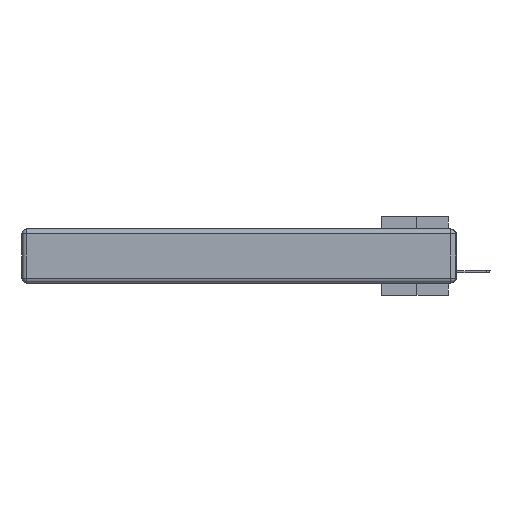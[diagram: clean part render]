
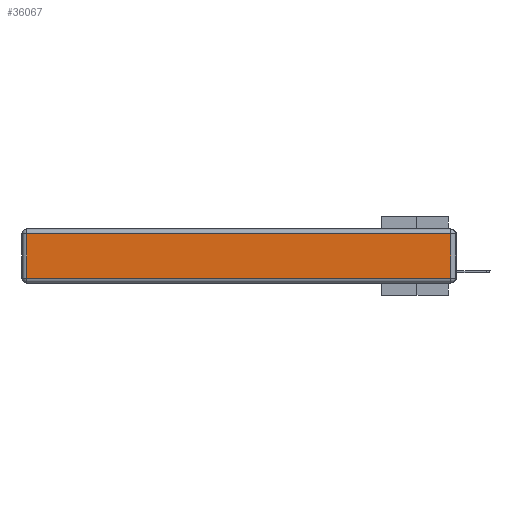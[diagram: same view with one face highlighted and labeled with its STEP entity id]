
A CAD part, left-side view. The second image highlights one B-rep face of the part: STEP entity #36067.
In plain terms, the highlighted planar face has unit normal (-1, 0, 0).
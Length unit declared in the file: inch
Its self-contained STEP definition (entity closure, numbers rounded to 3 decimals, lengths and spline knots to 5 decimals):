
#147 = LINE ( 'NONE', #37294, #10879 ) ;
#1068 = DIRECTION ( 'NONE',  ( 0., 0., -1. ) ) ;
#3771 = CARTESIAN_POINT ( 'NONE',  ( 0., 0.03, -0.343 ) ) ;
#5333 = ORIENTED_EDGE ( 'NONE', *, *, #14270, .T. ) ;
#7902 = CARTESIAN_POINT ( 'NONE',  ( 0., 0.03, -0.313 ) ) ;
#9978 = CARTESIAN_POINT ( 'NONE',  ( 0., 0., -0.313 ) ) ;
#10535 = ORIENTED_EDGE ( 'NONE', *, *, #18602, .T. ) ;
#10879 = VECTOR ( 'NONE', #1068, 39.37008 ) ;
#10918 = VECTOR ( 'NONE', #33425, 39.37008 ) ;
#13853 = ORIENTED_EDGE ( 'NONE', *, *, #25827, .T. ) ;
#14108 = VECTOR ( 'NONE', #34492, 39.37008 ) ;
#14225 = CARTESIAN_POINT ( 'NONE',  ( 0., 0.03, -0.03 ) ) ;
#14270 = EDGE_CURVE ( 'NONE', #38192, #15046, #147, .T. ) ;
#15046 = VERTEX_POINT ( 'NONE', #20763 ) ;
#15452 = LINE ( 'NONE', #22217, #14108 ) ;
#16089 = VERTEX_POINT ( 'NONE', #14225 ) ;
#17217 = VECTOR ( 'NONE', #21709, 39.37008 ) ;
#17984 = LINE ( 'NONE', #9978, #10918 ) ;
#18602 = EDGE_CURVE ( 'NONE', #15046, #23825, #17984, .T. ) ;
#19033 = LINE ( 'NONE', #3771, #17217 ) ;
#19239 = FACE_OUTER_BOUND ( 'NONE', #38708, .T. ) ;
#19801 = EDGE_CURVE ( 'NONE', #16089, #38192, #15452, .T. ) ;
#20763 = CARTESIAN_POINT ( 'NONE',  ( 0., 2.72, -0.313 ) ) ;
#21709 = DIRECTION ( 'NONE',  ( 0., 0., 1. ) ) ;
#22217 = CARTESIAN_POINT ( 'NONE',  ( 0., 2.75, -0.03 ) ) ;
#23164 = CARTESIAN_POINT ( 'NONE',  ( 0., 2.72, -0.03 ) ) ;
#23825 = VERTEX_POINT ( 'NONE', #7902 ) ;
#24840 = DIRECTION ( 'NONE',  ( -1., 0., 0. ) ) ;
#25827 = EDGE_CURVE ( 'NONE', #23825, #16089, #19033, .T. ) ;
#30732 = DIRECTION ( 'NONE',  ( 0., 0., 1. ) ) ;
#32532 = AXIS2_PLACEMENT_3D ( 'NONE', #36501, #24840, #30732 ) ;
#33425 = DIRECTION ( 'NONE',  ( 0., -1., 0. ) ) ;
#33757 = PLANE ( 'NONE',  #32532 ) ;
#34492 = DIRECTION ( 'NONE',  ( 0., 1., 0. ) ) ;
#35568 = ORIENTED_EDGE ( 'NONE', *, *, #19801, .T. ) ;
#36067 = ADVANCED_FACE ( 'NONE', ( #19239 ), #33757, .T. ) ;
#36501 = CARTESIAN_POINT ( 'NONE',  ( 0., 0., -0.343 ) ) ;
#37294 = CARTESIAN_POINT ( 'NONE',  ( 0., 2.72, -0.343 ) ) ;
#38192 = VERTEX_POINT ( 'NONE', #23164 ) ;
#38708 = EDGE_LOOP ( 'NONE', ( #10535, #13853, #35568, #5333 ) ) ;
